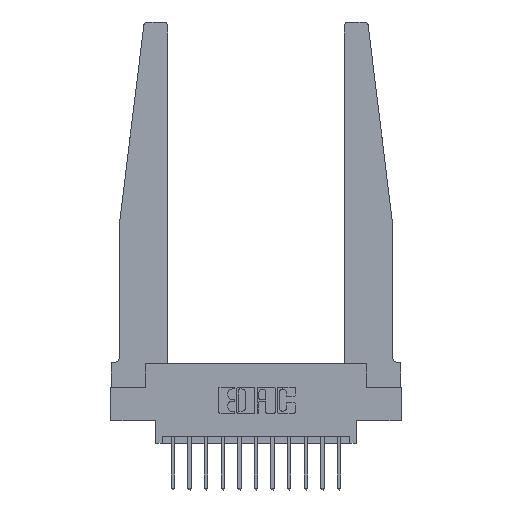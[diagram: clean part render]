
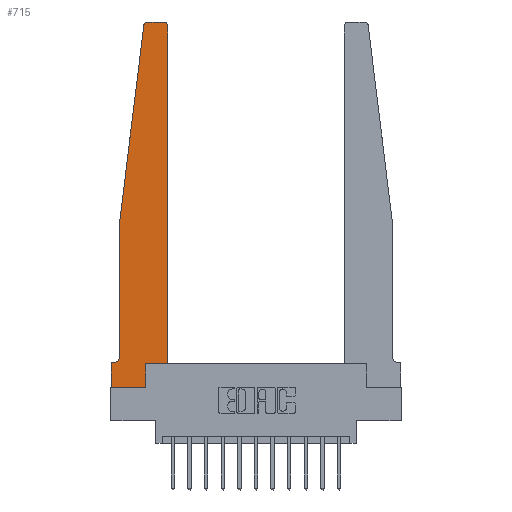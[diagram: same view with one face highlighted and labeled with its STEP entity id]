
A CAD part, top view. The second image highlights one B-rep face of the part: STEP entity #715.
In plain terms, the highlighted planar face has unit normal (0, 0, 1).
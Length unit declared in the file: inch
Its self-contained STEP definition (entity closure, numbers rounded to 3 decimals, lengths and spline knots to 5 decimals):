
#399 = EDGE_CURVE ( 'NONE', #12752, #3585, #13631, .T. ) ;
#635 = EDGE_CURVE ( 'NONE', #13616, #9811, #4225, .T. ) ;
#715 = ADVANCED_FACE ( 'NONE', ( #6774 ), #9499, .T. ) ;
#957 = VECTOR ( 'NONE', #11238, 39.37008 ) ;
#1050 = EDGE_CURVE ( 'NONE', #6946, #16126, #15384, .T. ) ;
#1054 = ORIENTED_EDGE ( 'NONE', *, *, #6326, .T. ) ;
#1268 = VECTOR ( 'NONE', #13523, 39.37008 ) ;
#1675 = CARTESIAN_POINT ( 'NONE',  ( 0., 0.1875, 0.37 ) ) ;
#2062 = DIRECTION ( 'NONE',  ( 1., 0., 0. ) ) ;
#2191 = ORIENTED_EDGE ( 'NONE', *, *, #15380, .T. ) ;
#2253 = DIRECTION ( 'NONE',  ( 0., -1., 0. ) ) ;
#2549 = LINE ( 'NONE', #4803, #5936 ) ;
#2735 = EDGE_CURVE ( 'NONE', #5913, #9413, #3087, .T. ) ;
#2828 = DIRECTION ( 'NONE',  ( 1., 0., 0. ) ) ;
#2914 = DIRECTION ( 'NONE',  ( 0., 0., 1. ) ) ;
#2932 = ORIENTED_EDGE ( 'NONE', *, *, #1050, .T. ) ;
#2933 = CARTESIAN_POINT ( 'NONE',  ( 0.395, 2.72, 0.37 ) ) ;
#3087 = CIRCLE ( 'NONE', #3610, 0.05 ) ;
#3278 = EDGE_CURVE ( 'NONE', #9413, #13616, #12682, .T. ) ;
#3564 = ORIENTED_EDGE ( 'NONE', *, *, #2735, .T. ) ;
#3585 = VERTEX_POINT ( 'NONE', #4760 ) ;
#3607 = VERTEX_POINT ( 'NONE', #12265 ) ;
#3610 = AXIS2_PLACEMENT_3D ( 'NONE', #14208, #6705, #15465 ) ;
#3883 = VERTEX_POINT ( 'NONE', #11725 ) ;
#4062 = CARTESIAN_POINT ( 'NONE',  ( 0.065, 0.1875, 0.37 ) ) ;
#4126 = EDGE_CURVE ( 'NONE', #3585, #6946, #4625, .T. ) ;
#4225 = LINE ( 'NONE', #11627, #13818 ) ;
#4489 = CARTESIAN_POINT ( 'NONE',  ( 0., 0., 0.37 ) ) ;
#4625 = LINE ( 'NONE', #4780, #1268 ) ;
#4700 = DIRECTION ( 'NONE',  ( 1., 0., 0. ) ) ;
#4760 = CARTESIAN_POINT ( 'NONE',  ( 0.425, 0.18, 0.37 ) ) ;
#4780 = CARTESIAN_POINT ( 'NONE',  ( 0.425, 0.18, 0.37 ) ) ;
#4803 = CARTESIAN_POINT ( 'NONE',  ( 0.065, 1.25, 0.37 ) ) ;
#5003 = CARTESIAN_POINT ( 'NONE',  ( 0.065, 1.25, 0.37 ) ) ;
#5327 = DIRECTION ( 'NONE',  ( -1., 0., 0. ) ) ;
#5554 = CARTESIAN_POINT ( 'NONE',  ( 0.425, 0.18, 0.37 ) ) ;
#5913 = VERTEX_POINT ( 'NONE', #11011 ) ;
#5936 = VECTOR ( 'NONE', #2253, 39.37008 ) ;
#5959 = VERTEX_POINT ( 'NONE', #8610 ) ;
#6041 = VECTOR ( 'NONE', #5327, 39.37008 ) ;
#6137 = EDGE_CURVE ( 'NONE', #5959, #13435, #10821, .T. ) ;
#6326 = EDGE_CURVE ( 'NONE', #9811, #3883, #14738, .T. ) ;
#6401 = EDGE_LOOP ( 'NONE', ( #8992, #13350, #2191, #15368, #3564, #8130, #15379, #1054, #9346, #7229, #12069, #2932 ) ) ;
#6460 = DIRECTION ( 'NONE',  ( 0., 0., 1. ) ) ;
#6579 = VECTOR ( 'NONE', #4700, 39.37008 ) ;
#6705 = DIRECTION ( 'NONE',  ( 0., 0., -1. ) ) ;
#6769 = EDGE_CURVE ( 'NONE', #3607, #5913, #2549, .T. ) ;
#6774 = FACE_OUTER_BOUND ( 'NONE', #6401, .T. ) ;
#6946 = VERTEX_POINT ( 'NONE', #12674 ) ;
#7229 = ORIENTED_EDGE ( 'NONE', *, *, #399, .T. ) ;
#7513 = CARTESIAN_POINT ( 'NONE',  ( 0.2605, 0.18, 0.37 ) ) ;
#7898 = LINE ( 'NONE', #7513, #11235 ) ;
#7950 = CARTESIAN_POINT ( 'NONE',  ( 0.25, 2.75, 0.37 ) ) ;
#8045 = AXIS2_PLACEMENT_3D ( 'NONE', #13960, #6460, #15442 ) ;
#8130 = ORIENTED_EDGE ( 'NONE', *, *, #3278, .T. ) ;
#8610 = CARTESIAN_POINT ( 'NONE',  ( 0.27653, 2.75, 0.37 ) ) ;
#8992 = ORIENTED_EDGE ( 'NONE', *, *, #12940, .T. ) ;
#9342 = DIRECTION ( 'NONE',  ( 1., 0., 0. ) ) ;
#9346 = ORIENTED_EDGE ( 'NONE', *, *, #9360, .T. ) ;
#9360 = EDGE_CURVE ( 'NONE', #3883, #12752, #7898, .T. ) ;
#9413 = VERTEX_POINT ( 'NONE', #15072 ) ;
#9414 = DIRECTION ( 'NONE',  ( 0., 0., 1. ) ) ;
#9484 = CARTESIAN_POINT ( 'NONE',  ( 0., 0.1875, 0.37 ) ) ;
#9499 = PLANE ( 'NONE',  #15037 ) ;
#9811 = VERTEX_POINT ( 'NONE', #12769 ) ;
#10821 = CIRCLE ( 'NONE', #8045, 0.03 ) ;
#10973 = DIRECTION ( 'NONE',  ( 0., -1., 0. ) ) ;
#11011 = CARTESIAN_POINT ( 'NONE',  ( 0.065, 0.2375, 0.37 ) ) ;
#11235 = VECTOR ( 'NONE', #16292, 39.37008 ) ;
#11238 = DIRECTION ( 'NONE',  ( -0.122, -0.992, 0. ) ) ;
#11408 = VECTOR ( 'NONE', #2062, 39.37008 ) ;
#11587 = CARTESIAN_POINT ( 'NONE',  ( 0.395, 2.75, 0.37 ) ) ;
#11627 = CARTESIAN_POINT ( 'NONE',  ( 0., 0., 0.37 ) ) ;
#11725 = CARTESIAN_POINT ( 'NONE',  ( 0.2605, 0., 0.37 ) ) ;
#12069 = ORIENTED_EDGE ( 'NONE', *, *, #4126, .T. ) ;
#12265 = CARTESIAN_POINT ( 'NONE',  ( 0.065, 1.25, 0.37 ) ) ;
#12323 = LINE ( 'NONE', #7950, #15662 ) ;
#12390 = CARTESIAN_POINT ( 'NONE',  ( 0.2605, 0.18, 0.37 ) ) ;
#12597 = CARTESIAN_POINT ( 'NONE',  ( 0.24675, 2.72367, 0.37 ) ) ;
#12674 = CARTESIAN_POINT ( 'NONE',  ( 0.425, 2.72, 0.37 ) ) ;
#12682 = LINE ( 'NONE', #4062, #6041 ) ;
#12752 = VERTEX_POINT ( 'NONE', #12390 ) ;
#12769 = CARTESIAN_POINT ( 'NONE',  ( 0., 0., 0.37 ) ) ;
#12940 = EDGE_CURVE ( 'NONE', #16126, #5959, #12323, .T. ) ;
#13350 = ORIENTED_EDGE ( 'NONE', *, *, #6137, .T. ) ;
#13435 = VERTEX_POINT ( 'NONE', #12597 ) ;
#13523 = DIRECTION ( 'NONE',  ( 0., 1., 0. ) ) ;
#13616 = VERTEX_POINT ( 'NONE', #1675 ) ;
#13631 = LINE ( 'NONE', #5554, #6579 ) ;
#13818 = VECTOR ( 'NONE', #10973, 39.37008 ) ;
#13872 = AXIS2_PLACEMENT_3D ( 'NONE', #2933, #2914, #2828 ) ;
#13960 = CARTESIAN_POINT ( 'NONE',  ( 0.27653, 2.72, 0.37 ) ) ;
#14208 = CARTESIAN_POINT ( 'NONE',  ( 0.015, 0.2375, 0.37 ) ) ;
#14738 = LINE ( 'NONE', #4489, #11408 ) ;
#15037 = AXIS2_PLACEMENT_3D ( 'NONE', #9484, #9414, #9342 ) ;
#15072 = CARTESIAN_POINT ( 'NONE',  ( 0.015, 0.1875, 0.37 ) ) ;
#15107 = LINE ( 'NONE', #5003, #957 ) ;
#15368 = ORIENTED_EDGE ( 'NONE', *, *, #6769, .T. ) ;
#15379 = ORIENTED_EDGE ( 'NONE', *, *, #635, .T. ) ;
#15380 = EDGE_CURVE ( 'NONE', #13435, #3607, #15107, .T. ) ;
#15384 = CIRCLE ( 'NONE', #13872, 0.03 ) ;
#15442 = DIRECTION ( 'NONE',  ( 1., 0., 0. ) ) ;
#15451 = DIRECTION ( 'NONE',  ( -1., 0., 0. ) ) ;
#15465 = DIRECTION ( 'NONE',  ( -1., 0., 0. ) ) ;
#15662 = VECTOR ( 'NONE', #15451, 39.37008 ) ;
#16126 = VERTEX_POINT ( 'NONE', #11587 ) ;
#16292 = DIRECTION ( 'NONE',  ( 0., 1., 0. ) ) ;
